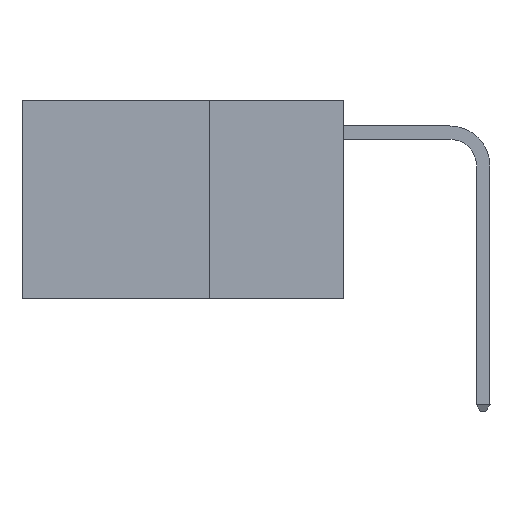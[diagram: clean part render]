
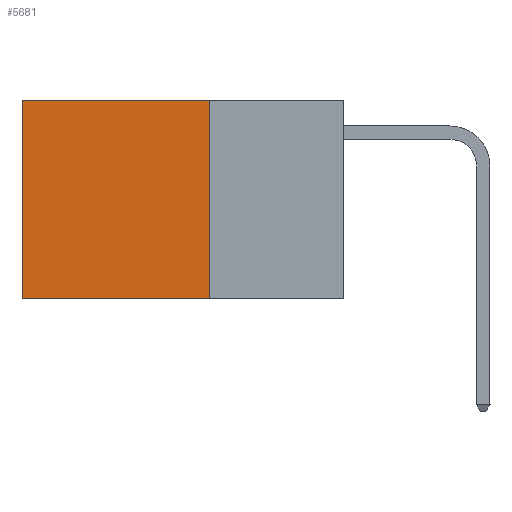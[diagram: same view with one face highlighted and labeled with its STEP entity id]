
A CAD part, left-side view. The second image highlights one B-rep face of the part: STEP entity #5681.
In plain terms, the highlighted planar face has unit normal (-1, 0, 0).
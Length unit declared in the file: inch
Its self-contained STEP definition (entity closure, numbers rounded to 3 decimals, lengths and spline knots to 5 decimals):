
#95 = DIRECTION ( 'NONE',  ( 0., 1., 0. ) ) ;
#558 = VERTEX_POINT ( 'NONE', #4760 ) ;
#628 = PLANE ( 'NONE',  #4499 ) ;
#1907 = LINE ( 'NONE', #13387, #3168 ) ;
#2085 = ORIENTED_EDGE ( 'NONE', *, *, #6234, .F. ) ;
#2952 = CARTESIAN_POINT ( 'NONE',  ( 0.2625, 0.25, -0.37 ) ) ;
#3168 = VECTOR ( 'NONE', #4036, 39.37008 ) ;
#3328 = ORIENTED_EDGE ( 'NONE', *, *, #3996, .F. ) ;
#3502 = DIRECTION ( 'NONE',  ( 0., 0., -1. ) ) ;
#3928 = CARTESIAN_POINT ( 'NONE',  ( 0.2625, 0.25, 0. ) ) ;
#3996 = EDGE_CURVE ( 'NONE', #5377, #9213, #1907, .T. ) ;
#4036 = DIRECTION ( 'NONE',  ( 0., 0., -1. ) ) ;
#4073 = VECTOR ( 'NONE', #5122, 39.37008 ) ;
#4264 = LINE ( 'NONE', #11615, #6322 ) ;
#4499 = AXIS2_PLACEMENT_3D ( 'NONE', #3928, #6905, #8892 ) ;
#4760 = CARTESIAN_POINT ( 'NONE',  ( 0.2625, 0.6, 0. ) ) ;
#5034 = CARTESIAN_POINT ( 'NONE',  ( 0.2625, 0.25, 0. ) ) ;
#5122 = DIRECTION ( 'NONE',  ( 0., 1., 0. ) ) ;
#5377 = VERTEX_POINT ( 'NONE', #9310 ) ;
#5681 = ADVANCED_FACE ( 'NONE', ( #13273 ), #628, .F. ) ;
#6234 = EDGE_CURVE ( 'NONE', #9213, #10428, #10169, .T. ) ;
#6322 = VECTOR ( 'NONE', #3502, 39.37008 ) ;
#6905 = DIRECTION ( 'NONE',  ( 1., 0., 0. ) ) ;
#7119 = VECTOR ( 'NONE', #95, 39.37008 ) ;
#7709 = CARTESIAN_POINT ( 'NONE',  ( 0.2625, 0.25, -0.37 ) ) ;
#8123 = EDGE_CURVE ( 'NONE', #5377, #558, #11235, .T. ) ;
#8222 = CARTESIAN_POINT ( 'NONE',  ( 0.2625, 0.6, -0.37 ) ) ;
#8892 = DIRECTION ( 'NONE',  ( 0., 0., -1. ) ) ;
#9213 = VERTEX_POINT ( 'NONE', #7709 ) ;
#9310 = CARTESIAN_POINT ( 'NONE',  ( 0.2625, 0.25, 0. ) ) ;
#10169 = LINE ( 'NONE', #2952, #4073 ) ;
#10428 = VERTEX_POINT ( 'NONE', #8222 ) ;
#11235 = LINE ( 'NONE', #5034, #7119 ) ;
#11615 = CARTESIAN_POINT ( 'NONE',  ( 0.2625, 0.6, 0. ) ) ;
#11733 = EDGE_CURVE ( 'NONE', #558, #10428, #4264, .T. ) ;
#11792 = EDGE_LOOP ( 'NONE', ( #11875, #2085, #3328, #12184 ) ) ;
#11875 = ORIENTED_EDGE ( 'NONE', *, *, #11733, .T. ) ;
#12184 = ORIENTED_EDGE ( 'NONE', *, *, #8123, .T. ) ;
#13273 = FACE_OUTER_BOUND ( 'NONE', #11792, .T. ) ;
#13387 = CARTESIAN_POINT ( 'NONE',  ( 0.2625, 0.25, 0. ) ) ;
